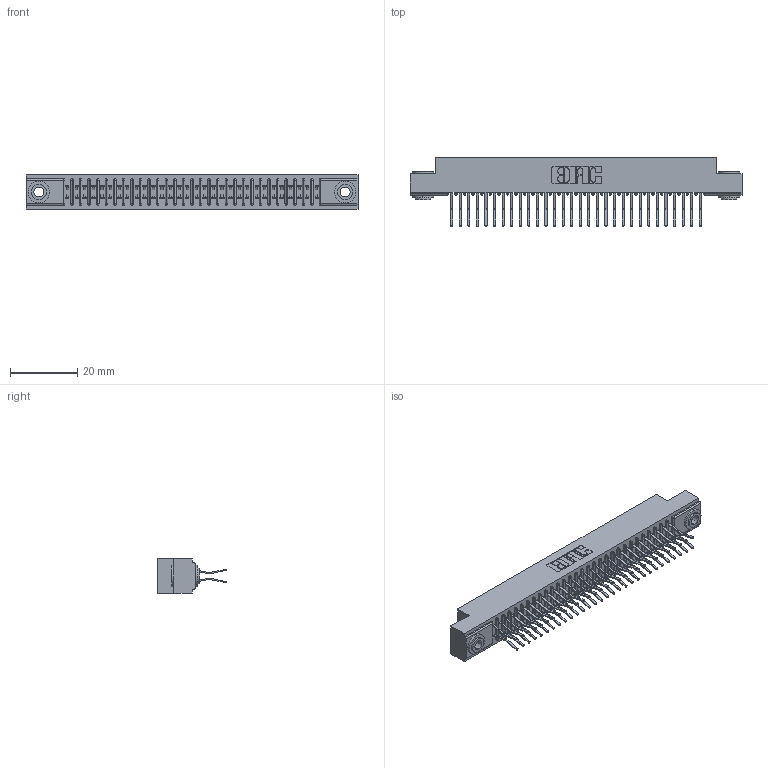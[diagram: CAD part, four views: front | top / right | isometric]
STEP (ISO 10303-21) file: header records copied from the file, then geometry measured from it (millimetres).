
FILE_DESCRIPTION (( 'STEP AP203' ), '1' );
FILE_NAME ('341-060-560-203.STEP', '2018-08-07T17:41:18', ( '' ), ( '' ), 'SwSTEP 2.0', 'SolidWorks 2016', '' );
FILE_SCHEMA (( 'CONFIG_CONTROL_DESIGN' ));
Length unit declared in the file: inch
Products named in the file (4): 345-250-002_345-250-002-102; 341 Part_.156 (3.96) Dia Mounting Holes; 341-060-560-203; 341-292-001_341-292-160
Assembly tree (63 placements, depth 2):
  341-060-560-203
    341 Part_.156 (3.96) Dia Mounting Holes
    341-292-001_341-292-160  x60
    345-250-002_345-250-002-102  x2
Bounding box: 98.42 x 20.37 x 10.16 mm (x, y, z)
Volume: 7318.5 mm3; surface area: 13300.8 mm2
Topology: 63 solids, 63 shells, 4368 faces, 12638 edges, 8198 vertices
Faces by surface type: plane 2492, cylinder 1748, sphere 62, torus 58, cone 8
Entity records: 39110 total; most frequent: CARTESIAN_POINT 6483, ORIENTED_EDGE 6432, DIRECTION 6320, EDGE_CURVE 3216, LINE 2570, VECTOR 2570, VERTEX_POINT 2038, AXIS2_PLACEMENT_3D 1875
